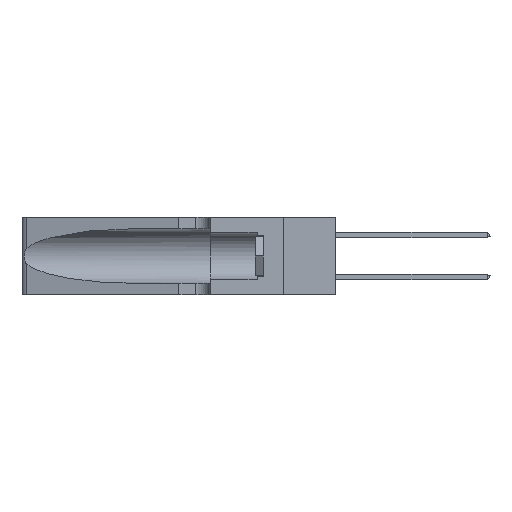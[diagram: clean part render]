
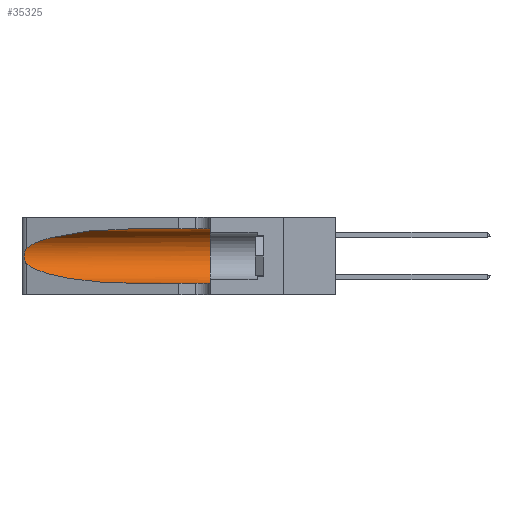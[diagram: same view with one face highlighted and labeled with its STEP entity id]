
A CAD part, left-side view. The second image highlights one B-rep face of the part: STEP entity #35325.
In plain terms, the highlighted cylindrical face has radius 3.308 mm (diameter 6.617 mm), a partial arc.
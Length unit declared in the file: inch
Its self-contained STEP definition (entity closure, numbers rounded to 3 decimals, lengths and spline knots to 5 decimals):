
#353 = CARTESIAN_POINT ( 'NONE',  ( 0.18966, 0.96281, 0.05475 ) ) ;
#2127 = CARTESIAN_POINT ( 'NONE',  ( 0.26018, 1.23835, 0.19895 ) ) ;
#2353 = CARTESIAN_POINT ( 'NONE',  ( 0.1305, 0.72297, 0.05475 ) ) ;
#4640 = VERTEX_POINT ( 'NONE', #24522 ) ;
#4934 = CARTESIAN_POINT ( 'NONE',  ( 0.18966, 0.96281, 0.31525 ) ) ;
#5179 = CARTESIAN_POINT ( 'NONE',  ( 0.1305, 0.35, 0.05475 ) ) ;
#5298 = CARTESIAN_POINT ( 'NONE',  ( 0.26075, 1.23896, 0.178 ) ) ;
#5615 = CARTESIAN_POINT ( 'NONE',  ( 0.1305, 0.35, 0.31525 ) ) ;
#6782 = DIRECTION ( 'NONE',  ( 0., -1., 0. ) ) ;
#8306 = CARTESIAN_POINT ( 'NONE',  ( 0.25487, 1.22718, 0.22369 ) ) ;
#8443 = CARTESIAN_POINT ( 'NONE',  ( 0.25856, 1.23593, 0.16098 ) ) ;
#8920 = CARTESIAN_POINT ( 'NONE',  ( 0.25487, 1.22718, 0.14631 ) ) ;
#10136 = FACE_OUTER_BOUND ( 'NONE', #16402, .T. ) ;
#10533 = VERTEX_POINT ( 'NONE', #5179 ) ;
#11256 = LINE ( 'NONE', #21350, #34613 ) ;
#11583 = CARTESIAN_POINT ( 'NONE',  ( 0.25639, 1.23186, 0.15144 ) ) ;
#12089 = ORIENTED_EDGE ( 'NONE', *, *, #25452, .F. ) ;
#12601 = EDGE_CURVE ( 'NONE', #4640, #19339, #28260, .T. ) ;
#12679 = DIRECTION ( 'NONE',  ( 0., 1., 0. ) ) ;
#12932 = CARTESIAN_POINT ( 'NONE',  ( 0.25487, 1.22718, 0.14631 ) ) ;
#13021 = DIRECTION ( 'NONE',  ( 0., 0., -1. ) ) ;
#13412 = CARTESIAN_POINT ( 'NONE',  ( 0.25487, 1.22718, 0.22369 ) ) ;
#13733 = ORIENTED_EDGE ( 'NONE', *, *, #22746, .T. ) ;
#14486 = CARTESIAN_POINT ( 'NONE',  ( 0.25487, 1.22718, 0.22369 ) ) ;
#14699 = CARTESIAN_POINT ( 'NONE',  ( 0.25487, 1.22718, 0.14631 ) ) ;
#15643 = EDGE_CURVE ( 'NONE', #34841, #30229, #16855, .T. ) ;
#16402 = EDGE_LOOP ( 'NONE', ( #32464, #35609, #26166, #13733, #12089, #20873 ) ) ;
#16855 =( BOUNDED_CURVE ( )  B_SPLINE_CURVE ( 3, ( #12932, #28166, #353, #34223 ),
 .UNSPECIFIED., .F., .T. ) 
 B_SPLINE_CURVE_WITH_KNOTS ( ( 4, 4 ),
 ( 3.44316, 4.71239 ),
 .UNSPECIFIED. ) 
 CURVE ( )  GEOMETRIC_REPRESENTATION_ITEM ( )  RATIONAL_B_SPLINE_CURVE ( ( 1., 0.87, 0.87, 1. ) ) 
 REPRESENTATION_ITEM ( '' )  );
#17401 = CYLINDRICAL_SURFACE ( 'NONE', #34035, 0.13025 ) ;
#17667 = CARTESIAN_POINT ( 'NONE',  ( 0.25639, 1.23184, 0.21858 ) ) ;
#19339 = VERTEX_POINT ( 'NONE', #13412 ) ;
#19655 = B_SPLINE_CURVE_WITH_KNOTS ( 'NONE', 3,
 ( #8306, #32768, #17667, #38820, #20727, #2127, #23799, #5298, #26859, #8443, #29890, #11583, #32899, #14699 ),
 .UNSPECIFIED., .F., .F.,
 ( 4, 2, 2, 2, 2, 2, 4 ),
 ( 0., 0.00027, 0.00053, 0.00107, 0.0016, 0.00187, 0.00214 ),
 .UNSPECIFIED. ) ;
#20727 = CARTESIAN_POINT ( 'NONE',  ( 0.25854, 1.2359, 0.20912 ) ) ;
#20873 = ORIENTED_EDGE ( 'NONE', *, *, #32916, .F. ) ;
#21153 = VECTOR ( 'NONE', #30342, 39.37008 ) ;
#21350 = CARTESIAN_POINT ( 'NONE',  ( 0.1305, 1.61858, 0.05475 ) ) ;
#22171 = CARTESIAN_POINT ( 'NONE',  ( 0.1305, 1.61858, 0.185 ) ) ;
#22746 = EDGE_CURVE ( 'NONE', #30229, #10533, #11256, .T. ) ;
#23799 = CARTESIAN_POINT ( 'NONE',  ( 0.26075, 1.23896, 0.19203 ) ) ;
#24522 = CARTESIAN_POINT ( 'NONE',  ( 0.1305, 0.72297, 0.31525 ) ) ;
#24593 = AXIS2_PLACEMENT_3D ( 'NONE', #30955, #12679, #33984 ) ;
#25452 = EDGE_CURVE ( 'NONE', #26044, #10533, #35317, .T. ) ;
#26044 = VERTEX_POINT ( 'NONE', #5615 ) ;
#26166 = ORIENTED_EDGE ( 'NONE', *, *, #15643, .T. ) ;
#26859 = CARTESIAN_POINT ( 'NONE',  ( 0.26017, 1.23833, 0.17102 ) ) ;
#28166 = CARTESIAN_POINT ( 'NONE',  ( 0.2373, 1.15595, 0.08982 ) ) ;
#28260 =( BOUNDED_CURVE ( )  B_SPLINE_CURVE ( 3, ( #35592, #4934, #32696, #14486 ),
 .UNSPECIFIED., .F., .F. ) 
 B_SPLINE_CURVE_WITH_KNOTS ( ( 4, 4 ),
 ( 1.5708, 2.84003 ),
 .UNSPECIFIED. ) 
 CURVE ( )  GEOMETRIC_REPRESENTATION_ITEM ( )  RATIONAL_B_SPLINE_CURVE ( ( 1., 0.87, 0.87, 1. ) ) 
 REPRESENTATION_ITEM ( '' )  );
#29528 = EDGE_CURVE ( 'NONE', #19339, #34841, #19655, .T. ) ;
#29890 = CARTESIAN_POINT ( 'NONE',  ( 0.25789, 1.23486, 0.15765 ) ) ;
#30173 = LINE ( 'NONE', #39281, #21153 ) ;
#30229 = VERTEX_POINT ( 'NONE', #2353 ) ;
#30342 = DIRECTION ( 'NONE',  ( 0., -1., 0. ) ) ;
#30491 = DIRECTION ( 'NONE',  ( 0., -1., 0. ) ) ;
#30955 = CARTESIAN_POINT ( 'NONE',  ( 0.1305, 0.35, 0.185 ) ) ;
#32464 = ORIENTED_EDGE ( 'NONE', *, *, #12601, .T. ) ;
#32696 = CARTESIAN_POINT ( 'NONE',  ( 0.2373, 1.15595, 0.28018 ) ) ;
#32768 = CARTESIAN_POINT ( 'NONE',  ( 0.25555, 1.22994, 0.2215 ) ) ;
#32899 = CARTESIAN_POINT ( 'NONE',  ( 0.25555, 1.22993, 0.14849 ) ) ;
#32916 = EDGE_CURVE ( 'NONE', #4640, #26044, #30173, .T. ) ;
#33984 = DIRECTION ( 'NONE',  ( 0., 0., 1. ) ) ;
#34035 = AXIS2_PLACEMENT_3D ( 'NONE', #22171, #6782, #13021 ) ;
#34223 = CARTESIAN_POINT ( 'NONE',  ( 0.1305, 0.72297, 0.05475 ) ) ;
#34613 = VECTOR ( 'NONE', #30491, 39.37008 ) ;
#34841 = VERTEX_POINT ( 'NONE', #8920 ) ;
#35317 = CIRCLE ( 'NONE', #24593, 0.13025 ) ;
#35325 = ADVANCED_FACE ( 'NONE', ( #10136 ), #17401, .F. ) ;
#35592 = CARTESIAN_POINT ( 'NONE',  ( 0.1305, 0.72297, 0.31525 ) ) ;
#35609 = ORIENTED_EDGE ( 'NONE', *, *, #29528, .T. ) ;
#38820 = CARTESIAN_POINT ( 'NONE',  ( 0.25787, 1.23484, 0.2124 ) ) ;
#39281 = CARTESIAN_POINT ( 'NONE',  ( 0.1305, 1.61858, 0.31525 ) ) ;
